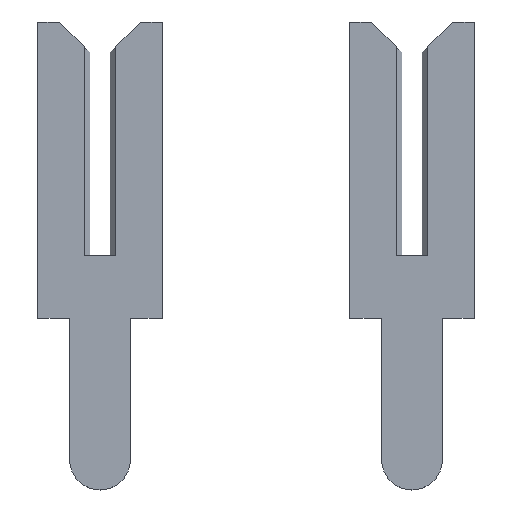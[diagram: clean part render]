
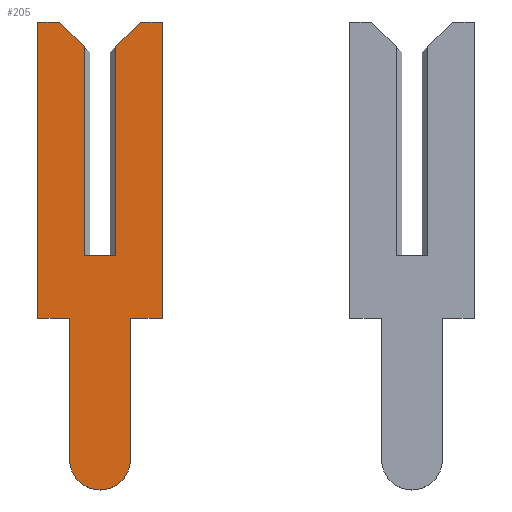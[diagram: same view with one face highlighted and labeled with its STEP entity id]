
A CAD part, top view. The second image highlights one B-rep face of the part: STEP entity #205.
In plain terms, the highlighted face is planar.
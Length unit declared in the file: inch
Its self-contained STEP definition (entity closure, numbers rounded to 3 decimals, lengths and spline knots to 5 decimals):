
#6 = EDGE_CURVE ( 'NONE', #419, #447, #120, .T. ) ;
#7 = VECTOR ( 'NONE', #653, 39.37008 ) ;
#11 = DIRECTION ( 'NONE',  ( 1., 0., 0. ) ) ;
#33 = LINE ( 'NONE', #486, #152 ) ;
#46 = ORIENTED_EDGE ( 'NONE', *, *, #331, .T. ) ;
#47 = EDGE_CURVE ( 'NONE', #123, #664, #394, .T. ) ;
#50 = CARTESIAN_POINT ( 'NONE',  ( -0.01, 0.15, -0.026 ) ) ;
#53 = CARTESIAN_POINT ( 'NONE',  ( -0.01, -0.04, 0.0195 ) ) ;
#72 = EDGE_CURVE ( 'NONE', #279, #649, #373, .T. ) ;
#75 = EDGE_CURVE ( 'NONE', #504, #681, #594, .T. ) ;
#82 = CARTESIAN_POINT ( 'NONE',  ( -0.01, -0.04, -0.04 ) ) ;
#93 = EDGE_CURVE ( 'NONE', #664, #278, #201, .T. ) ;
#98 = ORIENTED_EDGE ( 'NONE', *, *, #185, .F. ) ;
#101 = CARTESIAN_POINT ( 'NONE',  ( -0.01, -0.1305, 0.0195 ) ) ;
#106 = VERTEX_POINT ( 'NONE', #207 ) ;
#111 = VECTOR ( 'NONE', #274, 39.37008 ) ;
#113 = DIRECTION ( 'NONE',  ( 0., 0., 1. ) ) ;
#120 = LINE ( 'NONE', #390, #450 ) ;
#123 = VERTEX_POINT ( 'NONE', #53 ) ;
#130 = DIRECTION ( 'NONE',  ( 0., -1., 0. ) ) ;
#133 = CARTESIAN_POINT ( 'NONE',  ( -0.01, 0., -0.01 ) ) ;
#137 = VECTOR ( 'NONE', #512, 39.37008 ) ;
#144 = CARTESIAN_POINT ( 'NONE',  ( -0.01, -0.1305, 0. ) ) ;
#145 = FACE_OUTER_BOUND ( 'NONE', #539, .T. ) ;
#147 = EDGE_CURVE ( 'NONE', #243, #123, #792, .T. ) ;
#150 = CARTESIAN_POINT ( 'NONE',  ( -0.01, 0., 0.0065 ) ) ;
#152 = VECTOR ( 'NONE', #688, 39.37008 ) ;
#156 = VERTEX_POINT ( 'NONE', #133 ) ;
#164 = VECTOR ( 'NONE', #113, 39.37008 ) ;
#177 = VECTOR ( 'NONE', #722, 39.37008 ) ;
#185 = EDGE_CURVE ( 'NONE', #671, #419, #646, .T. ) ;
#188 = VECTOR ( 'NONE', #212, 39.37008 ) ;
#201 = CIRCLE ( 'NONE', #666, 0.0195 ) ;
#205 = ADVANCED_FACE ( 'NONE', ( #145 ), #218, .F. ) ;
#207 = CARTESIAN_POINT ( 'NONE',  ( -0.01, 0.15, 0.04 ) ) ;
#212 = DIRECTION ( 'NONE',  ( 0., 0., -1. ) ) ;
#218 = PLANE ( 'NONE',  #693 ) ;
#221 = VECTOR ( 'NONE', #130, 39.37008 ) ;
#233 = ORIENTED_EDGE ( 'NONE', *, *, #239, .F. ) ;
#239 = EDGE_CURVE ( 'NONE', #681, #156, #456, .T. ) ;
#240 = CARTESIAN_POINT ( 'NONE',  ( -0.01, 0.134, -0.01 ) ) ;
#243 = VERTEX_POINT ( 'NONE', #467 ) ;
#245 = CARTESIAN_POINT ( 'NONE',  ( -0.01, 0.15, 0.026 ) ) ;
#264 = ORIENTED_EDGE ( 'NONE', *, *, #6, .F. ) ;
#272 = CARTESIAN_POINT ( 'NONE',  ( -0.01, -0.04, -0.0195 ) ) ;
#274 = DIRECTION ( 'NONE',  ( 0., 0., -1. ) ) ;
#278 = VERTEX_POINT ( 'NONE', #342 ) ;
#279 = VERTEX_POINT ( 'NONE', #672 ) ;
#286 = VECTOR ( 'NONE', #478, 39.37008 ) ;
#304 = VERTEX_POINT ( 'NONE', #549 ) ;
#311 = EDGE_CURVE ( 'NONE', #278, #671, #774, .T. ) ;
#315 = LINE ( 'NONE', #841, #137 ) ;
#322 = CARTESIAN_POINT ( 'NONE',  ( -0.01, -0.1305, 0. ) ) ;
#331 = EDGE_CURVE ( 'NONE', #279, #304, #33, .T. ) ;
#335 = CARTESIAN_POINT ( 'NONE',  ( -0.01, -0.04, 0.04 ) ) ;
#342 = CARTESIAN_POINT ( 'NONE',  ( -0.01, -0.1305, -0.0195 ) ) ;
#351 = LINE ( 'NONE', #50, #503 ) ;
#361 = ORIENTED_EDGE ( 'NONE', *, *, #75, .F. ) ;
#373 = LINE ( 'NONE', #528, #177 ) ;
#389 = CARTESIAN_POINT ( 'NONE',  ( -0.01, 0.1305, -0.0065 ) ) ;
#390 = CARTESIAN_POINT ( 'NONE',  ( -0.01, 0.15, -0.04 ) ) ;
#394 = LINE ( 'NONE', #620, #221 ) ;
#409 = EDGE_CURVE ( 'NONE', #156, #304, #410, .T. ) ;
#410 = LINE ( 'NONE', #150, #587 ) ;
#419 = VERTEX_POINT ( 'NONE', #82 ) ;
#428 = LINE ( 'NONE', #245, #164 ) ;
#433 = CARTESIAN_POINT ( 'NONE',  ( -0.01, -0.04, -0.0195 ) ) ;
#447 = VERTEX_POINT ( 'NONE', #817 ) ;
#450 = VECTOR ( 'NONE', #452, 39.37008 ) ;
#452 = DIRECTION ( 'NONE',  ( 0., 1., 0. ) ) ;
#456 = LINE ( 'NONE', #546, #286 ) ;
#467 = CARTESIAN_POINT ( 'NONE',  ( -0.01, -0.04, 0.04 ) ) ;
#478 = DIRECTION ( 'NONE',  ( 0., -1., 0. ) ) ;
#486 = CARTESIAN_POINT ( 'NONE',  ( -0.01, 0.15, 0.01 ) ) ;
#494 = DIRECTION ( 'NONE',  ( 0., 0., 1. ) ) ;
#503 = VECTOR ( 'NONE', #707, 39.37008 ) ;
#504 = VERTEX_POINT ( 'NONE', #767 ) ;
#509 = CARTESIAN_POINT ( 'NONE',  ( -0.01, 0.15, 0.026 ) ) ;
#512 = DIRECTION ( 'NONE',  ( 0., -1., 0. ) ) ;
#515 = ORIENTED_EDGE ( 'NONE', *, *, #311, .F. ) ;
#528 = CARTESIAN_POINT ( 'NONE',  ( -0.01, 0.1305, 0.0065 ) ) ;
#539 = EDGE_LOOP ( 'NONE', ( #46, #762, #233, #361, #763, #264, #98, #515, #692, #685, #589, #691, #747, #830 ) ) ;
#546 = CARTESIAN_POINT ( 'NONE',  ( -0.01, -0.1305, -0.01 ) ) ;
#549 = CARTESIAN_POINT ( 'NONE',  ( -0.01, 0., 0.01 ) ) ;
#587 = VECTOR ( 'NONE', #494, 39.37008 ) ;
#589 = ORIENTED_EDGE ( 'NONE', *, *, #147, .F. ) ;
#594 = LINE ( 'NONE', #389, #7 ) ;
#610 = DIRECTION ( 'NONE',  ( 0., 1., 0. ) ) ;
#612 = CARTESIAN_POINT ( 'NONE',  ( -0.01, -0.04, -0.04 ) ) ;
#620 = CARTESIAN_POINT ( 'NONE',  ( -0.01, -0.04, 0.0195 ) ) ;
#646 = LINE ( 'NONE', #612, #111 ) ;
#649 = VERTEX_POINT ( 'NONE', #509 ) ;
#653 = DIRECTION ( 'NONE',  ( 0., -0.707, 0.707 ) ) ;
#655 = DIRECTION ( 'NONE',  ( 0., 0., -1. ) ) ;
#664 = VERTEX_POINT ( 'NONE', #101 ) ;
#666 = AXIS2_PLACEMENT_3D ( 'NONE', #322, #848, #655 ) ;
#671 = VERTEX_POINT ( 'NONE', #433 ) ;
#672 = CARTESIAN_POINT ( 'NONE',  ( -0.01, 0.134, 0.01 ) ) ;
#681 = VERTEX_POINT ( 'NONE', #240 ) ;
#685 = ORIENTED_EDGE ( 'NONE', *, *, #47, .F. ) ;
#688 = DIRECTION ( 'NONE',  ( 0., -1., 0. ) ) ;
#691 = ORIENTED_EDGE ( 'NONE', *, *, #803, .F. ) ;
#692 = ORIENTED_EDGE ( 'NONE', *, *, #93, .F. ) ;
#693 = AXIS2_PLACEMENT_3D ( 'NONE', #144, #11, #737 ) ;
#707 = DIRECTION ( 'NONE',  ( 0., 0., 1. ) ) ;
#714 = EDGE_CURVE ( 'NONE', #447, #504, #351, .T. ) ;
#722 = DIRECTION ( 'NONE',  ( 0., 0.707, 0.707 ) ) ;
#737 = DIRECTION ( 'NONE',  ( 0., 0., -1. ) ) ;
#747 = ORIENTED_EDGE ( 'NONE', *, *, #784, .F. ) ;
#762 = ORIENTED_EDGE ( 'NONE', *, *, #409, .F. ) ;
#763 = ORIENTED_EDGE ( 'NONE', *, *, #714, .F. ) ;
#767 = CARTESIAN_POINT ( 'NONE',  ( -0.01, 0.15, -0.026 ) ) ;
#774 = LINE ( 'NONE', #272, #776 ) ;
#776 = VECTOR ( 'NONE', #610, 39.37008 ) ;
#784 = EDGE_CURVE ( 'NONE', #649, #106, #428, .T. ) ;
#792 = LINE ( 'NONE', #335, #188 ) ;
#803 = EDGE_CURVE ( 'NONE', #106, #243, #315, .T. ) ;
#817 = CARTESIAN_POINT ( 'NONE',  ( -0.01, 0.15, -0.04 ) ) ;
#830 = ORIENTED_EDGE ( 'NONE', *, *, #72, .F. ) ;
#841 = CARTESIAN_POINT ( 'NONE',  ( -0.01, 0.15, 0.04 ) ) ;
#848 = DIRECTION ( 'NONE',  ( 1., 0., 0. ) ) ;
